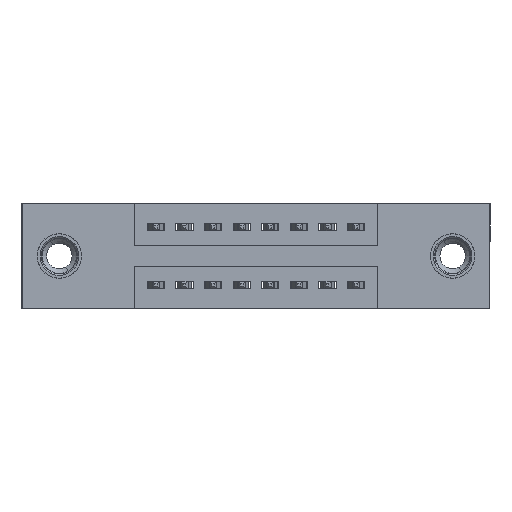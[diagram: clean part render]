
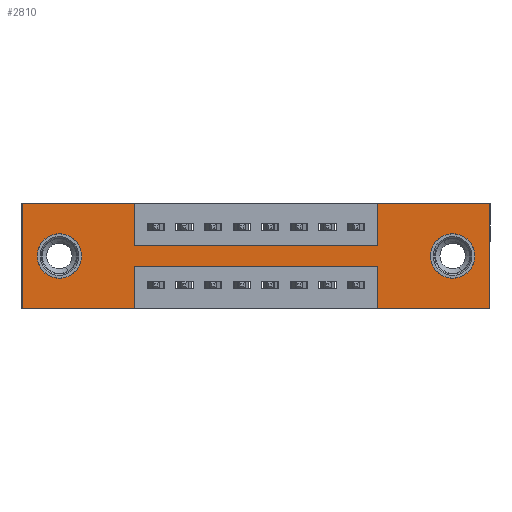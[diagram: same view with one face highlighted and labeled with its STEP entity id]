
A CAD part, front view. The second image highlights one B-rep face of the part: STEP entity #2810.
In plain terms, the highlighted planar face has unit normal (0, -1, 0).
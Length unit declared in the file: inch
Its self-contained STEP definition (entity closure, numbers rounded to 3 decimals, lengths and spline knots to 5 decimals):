
#306 = VERTEX_POINT ( 'NONE', #12372 ) ;
#315 = CARTESIAN_POINT ( 'NONE',  ( 1.2425, 0., -0.22 ) ) ;
#364 = VERTEX_POINT ( 'NONE', #8695 ) ;
#384 = VERTEX_POINT ( 'NONE', #9691 ) ;
#438 = EDGE_CURVE ( 'NONE', #8654, #3131, #11482, .T. ) ;
#674 = CARTESIAN_POINT ( 'NONE',  ( 1.2425, 0., 0. ) ) ;
#914 = LINE ( 'NONE', #8680, #11469 ) ;
#1182 = DIRECTION ( 'NONE',  ( 0., 1., 0. ) ) ;
#1437 = ORIENTED_EDGE ( 'NONE', *, *, #6374, .T. ) ;
#1841 = CARTESIAN_POINT ( 'NONE',  ( 1.2425, 0., 0. ) ) ;
#1964 = FACE_BOUND ( 'NONE', #11965, .T. ) ;
#2167 = DIRECTION ( 'NONE',  ( 0., 1., 0. ) ) ;
#2380 = CARTESIAN_POINT ( 'NONE',  ( 0., 0., 0. ) ) ;
#2428 = CARTESIAN_POINT ( 'NONE',  ( 1.635, 0., 0. ) ) ;
#2463 = CARTESIAN_POINT ( 'NONE',  ( 0., 0., 0. ) ) ;
#2513 = CARTESIAN_POINT ( 'NONE',  ( 1.635, 0., 0. ) ) ;
#2562 = CIRCLE ( 'NONE', #10334, 0.078 ) ;
#2650 = LINE ( 'NONE', #2463, #4575 ) ;
#2714 = VECTOR ( 'NONE', #7902, 39.37008 ) ;
#2788 = DIRECTION ( 'NONE',  ( -1., 0., 0. ) ) ;
#2810 = ADVANCED_FACE ( 'NONE', ( #1964, #11427, #15402 ), #13611, .T. ) ;
#3131 = VERTEX_POINT ( 'NONE', #6603 ) ;
#3271 = CARTESIAN_POINT ( 'NONE',  ( 0.3925, 0., -0.15 ) ) ;
#3351 = DIRECTION ( 'NONE',  ( 1., 0., 0. ) ) ;
#3364 = VERTEX_POINT ( 'NONE', #3271 ) ;
#3445 = ORIENTED_EDGE ( 'NONE', *, *, #7105, .T. ) ;
#3469 = EDGE_CURVE ( 'NONE', #8248, #306, #6109, .T. ) ;
#3626 = ORIENTED_EDGE ( 'NONE', *, *, #10126, .F. ) ;
#3845 = DIRECTION ( 'NONE',  ( 1., 0., 0. ) ) ;
#3928 = EDGE_LOOP ( 'NONE', ( #8143, #12665, #9995, #11317, #10394, #13091, #8087, #7417, #10815, #9341, #3626, #8096 ) ) ;
#4044 = EDGE_LOOP ( 'NONE', ( #1437, #3445 ) ) ;
#4416 = EDGE_CURVE ( 'NONE', #7196, #8290, #7757, .T. ) ;
#4420 = VECTOR ( 'NONE', #12109, 39.37008 ) ;
#4575 = VECTOR ( 'NONE', #4871, 39.37008 ) ;
#4818 = CARTESIAN_POINT ( 'NONE',  ( 0.13, 0., -0.185 ) ) ;
#4832 = DIRECTION ( 'NONE',  ( 0., 0., -1. ) ) ;
#4871 = DIRECTION ( 'NONE',  ( 1., 0., 0. ) ) ;
#4937 = CARTESIAN_POINT ( 'NONE',  ( 1.505, 0., -0.185 ) ) ;
#5037 = CARTESIAN_POINT ( 'NONE',  ( 1.635, 0., -0.37 ) ) ;
#5145 = LINE ( 'NONE', #14212, #12300 ) ;
#5187 = VECTOR ( 'NONE', #8500, 39.37008 ) ;
#5211 = CARTESIAN_POINT ( 'NONE',  ( 0., 0., 0. ) ) ;
#5218 = DIRECTION ( 'NONE',  ( 0., 0., -1. ) ) ;
#5230 = AXIS2_PLACEMENT_3D ( 'NONE', #4937, #8428, #14623 ) ;
#5454 = VERTEX_POINT ( 'NONE', #6229 ) ;
#5562 = LINE ( 'NONE', #12896, #2714 ) ;
#5584 = DIRECTION ( 'NONE',  ( 0., 0., -1. ) ) ;
#5624 = CIRCLE ( 'NONE', #9806, 0.078 ) ;
#5726 = VERTEX_POINT ( 'NONE', #9096 ) ;
#5788 = LINE ( 'NONE', #6694, #13915 ) ;
#6018 = CARTESIAN_POINT ( 'NONE',  ( 0.13, 0., -0.185 ) ) ;
#6091 = DIRECTION ( 'NONE',  ( 0., 0., 1. ) ) ;
#6109 = LINE ( 'NONE', #14420, #4420 ) ;
#6229 = CARTESIAN_POINT ( 'NONE',  ( 0.13, 0., -0.107 ) ) ;
#6370 = DIRECTION ( 'NONE',  ( 0., -1., 0. ) ) ;
#6374 = EDGE_CURVE ( 'NONE', #5454, #384, #12827, .T. ) ;
#6603 = CARTESIAN_POINT ( 'NONE',  ( 0.3925, 0., -0.22 ) ) ;
#6694 = CARTESIAN_POINT ( 'NONE',  ( 0.3925, 0., 0. ) ) ;
#6751 = ORIENTED_EDGE ( 'NONE', *, *, #7554, .T. ) ;
#6823 = CIRCLE ( 'NONE', #5230, 0.078 ) ;
#6986 = VERTEX_POINT ( 'NONE', #2428 ) ;
#7057 = EDGE_CURVE ( 'NONE', #14679, #5726, #13000, .T. ) ;
#7105 = EDGE_CURVE ( 'NONE', #384, #5454, #2562, .T. ) ;
#7196 = VERTEX_POINT ( 'NONE', #7570 ) ;
#7271 = DIRECTION ( 'NONE',  ( 0., 0., -1. ) ) ;
#7293 = EDGE_CURVE ( 'NONE', #8328, #13196, #914, .T. ) ;
#7299 = VECTOR ( 'NONE', #3845, 39.37008 ) ;
#7417 = ORIENTED_EDGE ( 'NONE', *, *, #11605, .F. ) ;
#7554 = EDGE_CURVE ( 'NONE', #364, #7638, #5624, .T. ) ;
#7570 = CARTESIAN_POINT ( 'NONE',  ( 1.2425, 0., -0.15 ) ) ;
#7638 = VERTEX_POINT ( 'NONE', #10374 ) ;
#7757 = LINE ( 'NONE', #674, #11754 ) ;
#7844 = AXIS2_PLACEMENT_3D ( 'NONE', #11281, #6370, #5218 ) ;
#7902 = DIRECTION ( 'NONE',  ( 0., 0., 1. ) ) ;
#7913 = LINE ( 'NONE', #11373, #8845 ) ;
#8087 = ORIENTED_EDGE ( 'NONE', *, *, #4416, .F. ) ;
#8096 = ORIENTED_EDGE ( 'NONE', *, *, #7293, .F. ) ;
#8143 = ORIENTED_EDGE ( 'NONE', *, *, #12151, .F. ) ;
#8243 = EDGE_CURVE ( 'NONE', #5726, #3364, #5788, .T. ) ;
#8248 = VERTEX_POINT ( 'NONE', #5037 ) ;
#8290 = VERTEX_POINT ( 'NONE', #1841 ) ;
#8328 = VERTEX_POINT ( 'NONE', #10290 ) ;
#8363 = VECTOR ( 'NONE', #7271, 39.37008 ) ;
#8428 = DIRECTION ( 'NONE',  ( 0., 1., 0. ) ) ;
#8500 = DIRECTION ( 'NONE',  ( 0., 0., 1. ) ) ;
#8602 = CARTESIAN_POINT ( 'NONE',  ( 0., 0., -0.37 ) ) ;
#8654 = VERTEX_POINT ( 'NONE', #315 ) ;
#8680 = CARTESIAN_POINT ( 'NONE',  ( 0., 0., -0.37 ) ) ;
#8695 = CARTESIAN_POINT ( 'NONE',  ( 1.505, 0., -0.107 ) ) ;
#8845 = VECTOR ( 'NONE', #5584, 39.37008 ) ;
#9096 = CARTESIAN_POINT ( 'NONE',  ( 0.3925, 0., 0. ) ) ;
#9159 = EDGE_CURVE ( 'NONE', #6986, #8248, #14847, .T. ) ;
#9302 = EDGE_CURVE ( 'NONE', #306, #8654, #5562, .T. ) ;
#9341 = ORIENTED_EDGE ( 'NONE', *, *, #7057, .F. ) ;
#9608 = CARTESIAN_POINT ( 'NONE',  ( 1.505, 0., -0.185 ) ) ;
#9631 = DIRECTION ( 'NONE',  ( 0., 0., 1. ) ) ;
#9685 = AXIS2_PLACEMENT_3D ( 'NONE', #6018, #1182, #9631 ) ;
#9691 = CARTESIAN_POINT ( 'NONE',  ( 0.13, 0., -0.263 ) ) ;
#9806 = AXIS2_PLACEMENT_3D ( 'NONE', #9608, #15511, #4832 ) ;
#9876 = LINE ( 'NONE', #2380, #5187 ) ;
#9995 = ORIENTED_EDGE ( 'NONE', *, *, #9302, .F. ) ;
#10126 = EDGE_CURVE ( 'NONE', #13196, #14679, #9876, .T. ) ;
#10290 = CARTESIAN_POINT ( 'NONE',  ( 0.3925, 0., -0.37 ) ) ;
#10334 = AXIS2_PLACEMENT_3D ( 'NONE', #4818, #2167, #13175 ) ;
#10374 = CARTESIAN_POINT ( 'NONE',  ( 1.505, 0., -0.263 ) ) ;
#10394 = ORIENTED_EDGE ( 'NONE', *, *, #9159, .F. ) ;
#10815 = ORIENTED_EDGE ( 'NONE', *, *, #8243, .F. ) ;
#11281 = CARTESIAN_POINT ( 'NONE',  ( 0., 0., -0.37 ) ) ;
#11317 = ORIENTED_EDGE ( 'NONE', *, *, #3469, .F. ) ;
#11373 = CARTESIAN_POINT ( 'NONE',  ( 0.3925, 0., -0.37 ) ) ;
#11427 = FACE_BOUND ( 'NONE', #4044, .T. ) ;
#11469 = VECTOR ( 'NONE', #15215, 39.37008 ) ;
#11482 = LINE ( 'NONE', #15173, #13740 ) ;
#11605 = EDGE_CURVE ( 'NONE', #3364, #7196, #5145, .T. ) ;
#11754 = VECTOR ( 'NONE', #6091, 39.37008 ) ;
#11965 = EDGE_LOOP ( 'NONE', ( #6751, #15400 ) ) ;
#12109 = DIRECTION ( 'NONE',  ( -1., 0., 0. ) ) ;
#12151 = EDGE_CURVE ( 'NONE', #3131, #8328, #7913, .T. ) ;
#12300 = VECTOR ( 'NONE', #3351, 39.37008 ) ;
#12372 = CARTESIAN_POINT ( 'NONE',  ( 1.2425, 0., -0.37 ) ) ;
#12665 = ORIENTED_EDGE ( 'NONE', *, *, #438, .F. ) ;
#12827 = CIRCLE ( 'NONE', #9685, 0.078 ) ;
#12896 = CARTESIAN_POINT ( 'NONE',  ( 1.2425, 0., -0.37 ) ) ;
#13000 = LINE ( 'NONE', #5211, #7299 ) ;
#13091 = ORIENTED_EDGE ( 'NONE', *, *, #15621, .F. ) ;
#13175 = DIRECTION ( 'NONE',  ( 0., 0., 1. ) ) ;
#13196 = VERTEX_POINT ( 'NONE', #8602 ) ;
#13611 = PLANE ( 'NONE',  #7844 ) ;
#13740 = VECTOR ( 'NONE', #2788, 39.37008 ) ;
#13880 = CARTESIAN_POINT ( 'NONE',  ( 0., 0., 0. ) ) ;
#13915 = VECTOR ( 'NONE', #15064, 39.37008 ) ;
#14212 = CARTESIAN_POINT ( 'NONE',  ( 0.3925, 0., -0.15 ) ) ;
#14420 = CARTESIAN_POINT ( 'NONE',  ( 0., 0., -0.37 ) ) ;
#14623 = DIRECTION ( 'NONE',  ( 0., 0., -1. ) ) ;
#14679 = VERTEX_POINT ( 'NONE', #13880 ) ;
#14847 = LINE ( 'NONE', #2513, #8363 ) ;
#14994 = EDGE_CURVE ( 'NONE', #7638, #364, #6823, .T. ) ;
#15064 = DIRECTION ( 'NONE',  ( 0., 0., -1. ) ) ;
#15173 = CARTESIAN_POINT ( 'NONE',  ( 0.3925, 0., -0.22 ) ) ;
#15215 = DIRECTION ( 'NONE',  ( -1., 0., 0. ) ) ;
#15400 = ORIENTED_EDGE ( 'NONE', *, *, #14994, .T. ) ;
#15402 = FACE_OUTER_BOUND ( 'NONE', #3928, .T. ) ;
#15511 = DIRECTION ( 'NONE',  ( 0., 1., 0. ) ) ;
#15621 = EDGE_CURVE ( 'NONE', #8290, #6986, #2650, .T. ) ;
